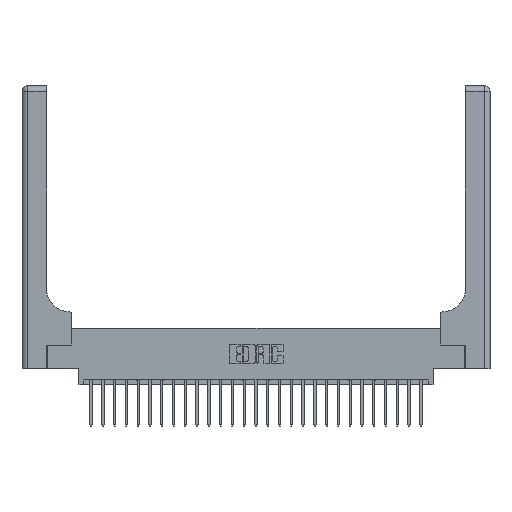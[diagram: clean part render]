
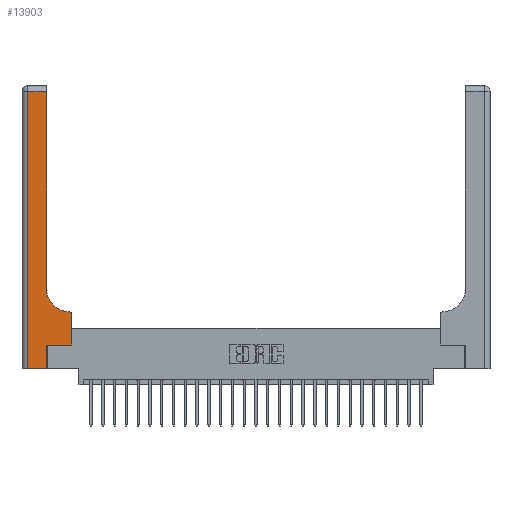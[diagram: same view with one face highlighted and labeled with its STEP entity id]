
A CAD part, top view. The second image highlights one B-rep face of the part: STEP entity #13903.
In plain terms, the highlighted planar face has unit normal (0, 0, 1).
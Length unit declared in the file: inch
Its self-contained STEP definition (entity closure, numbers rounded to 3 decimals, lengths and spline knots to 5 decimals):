
#841 = DIRECTION ( 'NONE',  ( 0., 0., -1. ) ) ;
#932 = EDGE_CURVE ( 'NONE', #9805, #8859, #15988, .T. ) ;
#1508 = DIRECTION ( 'NONE',  ( 0., 1., 0. ) ) ;
#1688 = ORIENTED_EDGE ( 'NONE', *, *, #3159, .T. ) ;
#1943 = CARTESIAN_POINT ( 'NONE',  ( 0.51, 0.85, 0.37 ) ) ;
#2303 = CARTESIAN_POINT ( 'NONE',  ( 0.26, 0.6, 0.37 ) ) ;
#2459 = EDGE_CURVE ( 'NONE', #18059, #11454, #25735, .T. ) ;
#2632 = CARTESIAN_POINT ( 'NONE',  ( 0.06, 0., 0.37 ) ) ;
#2944 = VERTEX_POINT ( 'NONE', #12461 ) ;
#3159 = EDGE_CURVE ( 'NONE', #7780, #2944, #5459, .T. ) ;
#3188 = EDGE_CURVE ( 'NONE', #23074, #11091, #5329, .T. ) ;
#3759 = CARTESIAN_POINT ( 'NONE',  ( 0.265, 0., 0.37 ) ) ;
#4317 = DIRECTION ( 'NONE',  ( -1., 0., 0. ) ) ;
#4491 = ORIENTED_EDGE ( 'NONE', *, *, #2459, .T. ) ;
#4670 = VECTOR ( 'NONE', #9955, 39.37008 ) ;
#5256 = VECTOR ( 'NONE', #7736, 39.37008 ) ;
#5329 = LINE ( 'NONE', #19678, #5256 ) ;
#5446 = AXIS2_PLACEMENT_3D ( 'NONE', #13320, #841, #17061 ) ;
#5459 = LINE ( 'NONE', #24190, #12266 ) ;
#6500 = LINE ( 'NONE', #6763, #13003 ) ;
#6700 = EDGE_CURVE ( 'NONE', #11454, #9805, #20259, .T. ) ;
#6723 = FACE_OUTER_BOUND ( 'NONE', #8990, .T. ) ;
#6763 = CARTESIAN_POINT ( 'NONE',  ( 0., 2.94, 0.37 ) ) ;
#6858 = PLANE ( 'NONE',  #5446 ) ;
#7342 = DIRECTION ( 'NONE',  ( 0., 1., 0. ) ) ;
#7509 = DIRECTION ( 'NONE',  ( 0., -1., 0. ) ) ;
#7736 = DIRECTION ( 'NONE',  ( 0., 1., 0. ) ) ;
#7780 = VERTEX_POINT ( 'NONE', #20054 ) ;
#8374 = VECTOR ( 'NONE', #4317, 39.37008 ) ;
#8859 = VERTEX_POINT ( 'NONE', #12895 ) ;
#8990 = EDGE_LOOP ( 'NONE', ( #1688, #20855, #4491, #11620, #22939, #12857, #12356, #18489, #25566 ) ) ;
#9206 = EDGE_CURVE ( 'NONE', #2944, #18059, #6500, .T. ) ;
#9805 = VERTEX_POINT ( 'NONE', #3759 ) ;
#9955 = DIRECTION ( 'NONE',  ( 1., 0., 0. ) ) ;
#10673 = DIRECTION ( 'NONE',  ( -1., 0., 0. ) ) ;
#11091 = VERTEX_POINT ( 'NONE', #19629 ) ;
#11454 = VERTEX_POINT ( 'NONE', #2632 ) ;
#11620 = ORIENTED_EDGE ( 'NONE', *, *, #6700, .T. ) ;
#11663 = CARTESIAN_POINT ( 'NONE',  ( 0.528, 0.25, 0.37 ) ) ;
#11784 = LINE ( 'NONE', #24216, #25443 ) ;
#12266 = VECTOR ( 'NONE', #7342, 39.37008 ) ;
#12356 = ORIENTED_EDGE ( 'NONE', *, *, #3188, .T. ) ;
#12461 = CARTESIAN_POINT ( 'NONE',  ( 0.26, 2.94, 0.37 ) ) ;
#12857 = ORIENTED_EDGE ( 'NONE', *, *, #23027, .T. ) ;
#12895 = CARTESIAN_POINT ( 'NONE',  ( 0.265, 0.25, 0.37 ) ) ;
#13003 = VECTOR ( 'NONE', #10673, 39.37008 ) ;
#13320 = CARTESIAN_POINT ( 'NONE',  ( 0., 3., 0.37 ) ) ;
#13515 = CIRCLE ( 'NONE', #21623, 0.25 ) ;
#13903 = ADVANCED_FACE ( 'NONE', ( #6723 ), #6858, .F. ) ;
#14149 = DIRECTION ( 'NONE',  ( 0., 0., -1. ) ) ;
#15552 = VERTEX_POINT ( 'NONE', #20367 ) ;
#15988 = LINE ( 'NONE', #22118, #25492 ) ;
#16384 = CARTESIAN_POINT ( 'NONE',  ( 0., 0., 0.37 ) ) ;
#17061 = DIRECTION ( 'NONE',  ( -1., 0., 0. ) ) ;
#18059 = VERTEX_POINT ( 'NONE', #22022 ) ;
#18489 = ORIENTED_EDGE ( 'NONE', *, *, #24598, .T. ) ;
#19321 = CARTESIAN_POINT ( 'NONE',  ( 0.06, 3., 0.37 ) ) ;
#19629 = CARTESIAN_POINT ( 'NONE',  ( 0.528, 0.6, 0.37 ) ) ;
#19678 = CARTESIAN_POINT ( 'NONE',  ( 0.528, 0.25, 0.37 ) ) ;
#19958 = DIRECTION ( 'NONE',  ( 1., 0., 0. ) ) ;
#20054 = CARTESIAN_POINT ( 'NONE',  ( 0.26, 0.85, 0.37 ) ) ;
#20259 = LINE ( 'NONE', #16384, #4670 ) ;
#20367 = CARTESIAN_POINT ( 'NONE',  ( 0.51, 0.6, 0.37 ) ) ;
#20855 = ORIENTED_EDGE ( 'NONE', *, *, #9206, .T. ) ;
#21623 = AXIS2_PLACEMENT_3D ( 'NONE', #1943, #14149, #22039 ) ;
#22022 = CARTESIAN_POINT ( 'NONE',  ( 0.06, 2.94, 0.37 ) ) ;
#22039 = DIRECTION ( 'NONE',  ( 1., 0., 0. ) ) ;
#22118 = CARTESIAN_POINT ( 'NONE',  ( 0.265, 0., 0.37 ) ) ;
#22529 = LINE ( 'NONE', #2303, #8374 ) ;
#22939 = ORIENTED_EDGE ( 'NONE', *, *, #932, .T. ) ;
#23027 = EDGE_CURVE ( 'NONE', #8859, #23074, #11784, .T. ) ;
#23074 = VERTEX_POINT ( 'NONE', #11663 ) ;
#24099 = EDGE_CURVE ( 'NONE', #15552, #7780, #13515, .T. ) ;
#24190 = CARTESIAN_POINT ( 'NONE',  ( 0.26, 3., 0.37 ) ) ;
#24216 = CARTESIAN_POINT ( 'NONE',  ( 0.265, 0.25, 0.37 ) ) ;
#24598 = EDGE_CURVE ( 'NONE', #11091, #15552, #22529, .T. ) ;
#25398 = VECTOR ( 'NONE', #7509, 39.37008 ) ;
#25443 = VECTOR ( 'NONE', #19958, 39.37008 ) ;
#25492 = VECTOR ( 'NONE', #1508, 39.37008 ) ;
#25566 = ORIENTED_EDGE ( 'NONE', *, *, #24099, .T. ) ;
#25735 = LINE ( 'NONE', #19321, #25398 ) ;
